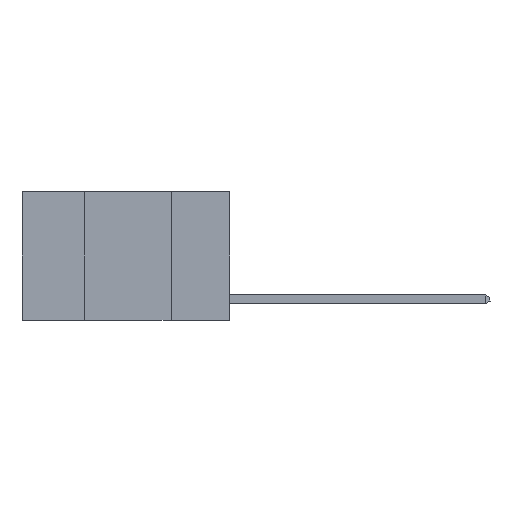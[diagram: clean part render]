
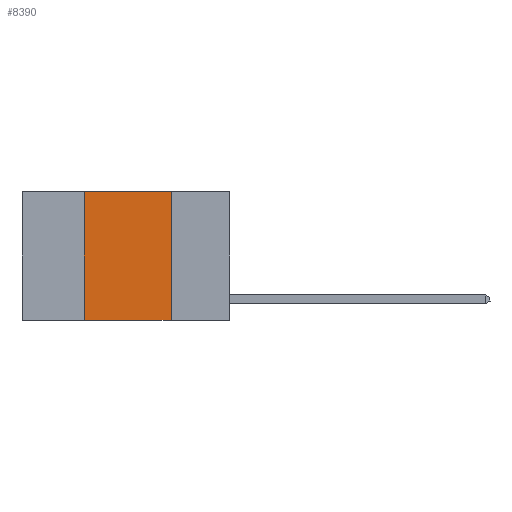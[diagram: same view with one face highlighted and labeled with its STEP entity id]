
A CAD part, left-side view. The second image highlights one B-rep face of the part: STEP entity #8390.
In plain terms, the highlighted planar face has unit normal (-1, 0, 0).
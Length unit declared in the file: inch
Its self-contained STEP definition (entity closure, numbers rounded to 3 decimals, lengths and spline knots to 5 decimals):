
#2326 = EDGE_CURVE ( 'NONE', #12393, #3161, #15439, .T. ) ;
#2329 = LINE ( 'NONE', #18145, #24503 ) ;
#2502 = EDGE_LOOP ( 'NONE', ( #25484, #3357, #4040, #16219 ) ) ;
#2702 = VECTOR ( 'NONE', #13836, 39.37008 ) ;
#3061 = CARTESIAN_POINT ( 'NONE',  ( 0., 0.42, -0.37 ) ) ;
#3161 = VERTEX_POINT ( 'NONE', #9021 ) ;
#3357 = ORIENTED_EDGE ( 'NONE', *, *, #2326, .F. ) ;
#4040 = ORIENTED_EDGE ( 'NONE', *, *, #5709, .F. ) ;
#4620 = EDGE_CURVE ( 'NONE', #3161, #22017, #19910, .T. ) ;
#4730 = DIRECTION ( 'NONE',  ( 1., 0., 0. ) ) ;
#5315 = VECTOR ( 'NONE', #23500, 39.37008 ) ;
#5333 = EDGE_CURVE ( 'NONE', #21329, #22017, #2329, .T. ) ;
#5709 = EDGE_CURVE ( 'NONE', #21329, #12393, #15877, .T. ) ;
#8390 = ADVANCED_FACE ( 'NONE', ( #21732 ), #21720, .F. ) ;
#8581 = CARTESIAN_POINT ( 'NONE',  ( 0., 0.6, 0. ) ) ;
#9021 = CARTESIAN_POINT ( 'NONE',  ( 0., 0.17, 0. ) ) ;
#11690 = CARTESIAN_POINT ( 'NONE',  ( 0., 0.17, 0. ) ) ;
#12393 = VERTEX_POINT ( 'NONE', #13849 ) ;
#13836 = DIRECTION ( 'NONE',  ( 0., 0., -1. ) ) ;
#13849 = CARTESIAN_POINT ( 'NONE',  ( 0., 0.42, 0. ) ) ;
#15439 = LINE ( 'NONE', #8581, #5315 ) ;
#15877 = LINE ( 'NONE', #17567, #26424 ) ;
#16219 = ORIENTED_EDGE ( 'NONE', *, *, #5333, .T. ) ;
#17567 = CARTESIAN_POINT ( 'NONE',  ( 0., 0.42, 0. ) ) ;
#17614 = CARTESIAN_POINT ( 'NONE',  ( 0., 0.6, 0. ) ) ;
#18145 = CARTESIAN_POINT ( 'NONE',  ( 0., 0.6, -0.37 ) ) ;
#19715 = DIRECTION ( 'NONE',  ( 0., 0., 1. ) ) ;
#19767 = DIRECTION ( 'NONE',  ( 0., 0., -1. ) ) ;
#19910 = LINE ( 'NONE', #11690, #2702 ) ;
#21329 = VERTEX_POINT ( 'NONE', #3061 ) ;
#21504 = AXIS2_PLACEMENT_3D ( 'NONE', #17614, #4730, #19767 ) ;
#21720 = PLANE ( 'NONE',  #21504 ) ;
#21732 = FACE_OUTER_BOUND ( 'NONE', #2502, .T. ) ;
#22017 = VERTEX_POINT ( 'NONE', #24751 ) ;
#23500 = DIRECTION ( 'NONE',  ( 0., -1., 0. ) ) ;
#24503 = VECTOR ( 'NONE', #26618, 39.37008 ) ;
#24751 = CARTESIAN_POINT ( 'NONE',  ( 0., 0.17, -0.37 ) ) ;
#25484 = ORIENTED_EDGE ( 'NONE', *, *, #4620, .F. ) ;
#26424 = VECTOR ( 'NONE', #19715, 39.37008 ) ;
#26618 = DIRECTION ( 'NONE',  ( 0., -1., 0. ) ) ;
